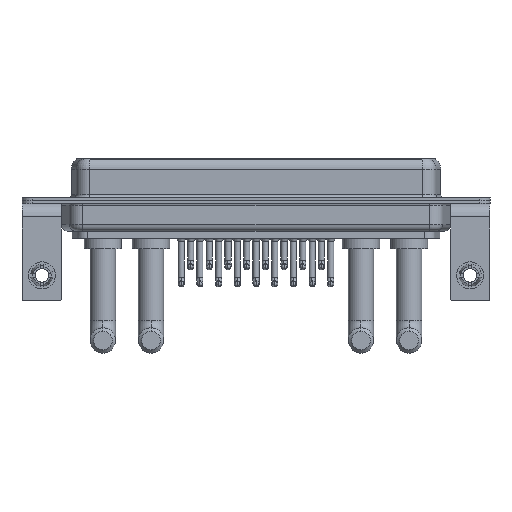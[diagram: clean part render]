
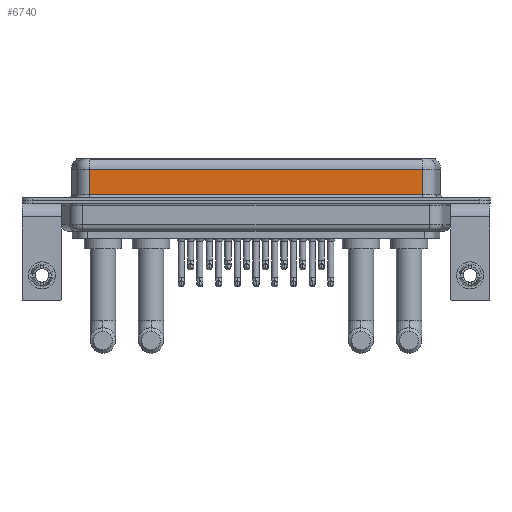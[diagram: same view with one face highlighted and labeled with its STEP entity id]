
A CAD part, front view. The second image highlights one B-rep face of the part: STEP entity #6740.
In plain terms, the highlighted planar face has unit normal (0, -1, 0).
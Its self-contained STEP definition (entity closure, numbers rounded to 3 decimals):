
#138 = VERTEX_POINT ( 'NONE', #17384 ) ;
#631 = CARTESIAN_POINT ( 'NONE',  ( 56.462, -3.95, 0.9 ) ) ;
#875 = CARTESIAN_POINT ( 'NONE',  ( 56.462, -3.95, 4.65 ) ) ;
#3666 = VECTOR ( 'NONE', #6549, 1000. ) ;
#4243 = PLANE ( 'NONE',  #10348 ) ;
#4371 = EDGE_CURVE ( 'NONE', #4490, #19376, #7095, .T. ) ;
#4490 = VERTEX_POINT ( 'NONE', #7468 ) ;
#5278 = DIRECTION ( 'NONE',  ( 0., 0., -1. ) ) ;
#6549 = DIRECTION ( 'NONE',  ( 0., 0., -1. ) ) ;
#6740 = ADVANCED_FACE ( 'NONE', ( #10200 ), #4243, .F. ) ;
#7095 = LINE ( 'NONE', #16401, #7396 ) ;
#7396 = VECTOR ( 'NONE', #23895, 1000. ) ;
#7468 = CARTESIAN_POINT ( 'NONE',  ( 7.038, -3.95, 0.9 ) ) ;
#7602 = CARTESIAN_POINT ( 'NONE',  ( 56.462, -3.95, 4.65 ) ) ;
#7812 = ORIENTED_EDGE ( 'NONE', *, *, #22216, .T. ) ;
#8748 = LINE ( 'NONE', #12850, #8770 ) ;
#8770 = VECTOR ( 'NONE', #5278, 1000. ) ;
#10200 = FACE_OUTER_BOUND ( 'NONE', #18863, .T. ) ;
#10348 = AXIS2_PLACEMENT_3D ( 'NONE', #19317, #15767, #19200 ) ;
#10727 = EDGE_CURVE ( 'NONE', #20765, #19376, #16312, .T. ) ;
#11258 = VECTOR ( 'NONE', #24275, 1000. ) ;
#12850 = CARTESIAN_POINT ( 'NONE',  ( 7.038, -3.95, 6.4 ) ) ;
#13958 = EDGE_CURVE ( 'NONE', #20765, #138, #18972, .T. ) ;
#14342 = CARTESIAN_POINT ( 'NONE',  ( 56.462, -3.95, 6.4 ) ) ;
#15767 = DIRECTION ( 'NONE',  ( 0., 1., 0. ) ) ;
#16312 = LINE ( 'NONE', #14342, #3666 ) ;
#16401 = CARTESIAN_POINT ( 'NONE',  ( 56.462, -3.95, 0.9 ) ) ;
#16809 = ORIENTED_EDGE ( 'NONE', *, *, #4371, .T. ) ;
#17384 = CARTESIAN_POINT ( 'NONE',  ( 7.038, -3.95, 4.65 ) ) ;
#18863 = EDGE_LOOP ( 'NONE', ( #24185, #21208, #7812, #16809 ) ) ;
#18972 = LINE ( 'NONE', #7602, #11258 ) ;
#19200 = DIRECTION ( 'NONE',  ( 0., 0., 1. ) ) ;
#19317 = CARTESIAN_POINT ( 'NONE',  ( 56.462, -3.95, 6.4 ) ) ;
#19376 = VERTEX_POINT ( 'NONE', #631 ) ;
#20765 = VERTEX_POINT ( 'NONE', #875 ) ;
#21208 = ORIENTED_EDGE ( 'NONE', *, *, #13958, .T. ) ;
#22216 = EDGE_CURVE ( 'NONE', #138, #4490, #8748, .T. ) ;
#23895 = DIRECTION ( 'NONE',  ( 1., 0., 0. ) ) ;
#24185 = ORIENTED_EDGE ( 'NONE', *, *, #10727, .F. ) ;
#24275 = DIRECTION ( 'NONE',  ( -1., 0., 0. ) ) ;
